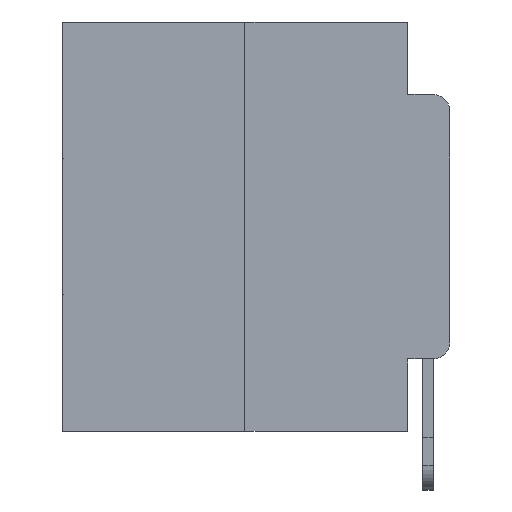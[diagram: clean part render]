
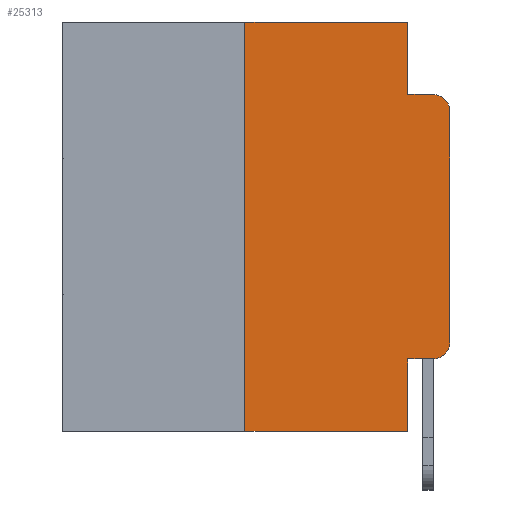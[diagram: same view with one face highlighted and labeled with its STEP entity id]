
A CAD part, left-side view. The second image highlights one B-rep face of the part: STEP entity #25313.
In plain terms, the highlighted planar face has unit normal (-1, 0, 0).
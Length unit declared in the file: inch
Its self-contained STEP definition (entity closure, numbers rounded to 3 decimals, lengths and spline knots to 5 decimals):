
#56 = CARTESIAN_POINT ( 'NONE',  ( 0., 0.25, -0.5 ) ) ;
#1165 = EDGE_CURVE ( 'NONE', #2305, #11096, #11929, .T. ) ;
#1232 = ORIENTED_EDGE ( 'NONE', *, *, #2636, .T. ) ;
#1287 = VECTOR ( 'NONE', #10315, 39.37008 ) ;
#1655 = CARTESIAN_POINT ( 'NONE',  ( 0., 0.051, -0.4115 ) ) ;
#1750 = CARTESIAN_POINT ( 'NONE',  ( 0., 0.051, -0.4115 ) ) ;
#1860 = ORIENTED_EDGE ( 'NONE', *, *, #25212, .T. ) ;
#2025 = AXIS2_PLACEMENT_3D ( 'NONE', #10923, #23818, #4348 ) ;
#2195 = CARTESIAN_POINT ( 'NONE',  ( 0., 0.473, 0. ) ) ;
#2305 = VERTEX_POINT ( 'NONE', #9074 ) ;
#2636 = EDGE_CURVE ( 'NONE', #25847, #20627, #27357, .T. ) ;
#2893 = EDGE_CURVE ( 'NONE', #9911, #21871, #22569, .T. ) ;
#3100 = CARTESIAN_POINT ( 'NONE',  ( 0., 0.02, -0.0885 ) ) ;
#3768 = VECTOR ( 'NONE', #12677, 39.37008 ) ;
#3935 = CARTESIAN_POINT ( 'NONE',  ( 0., 0.051, -0.5 ) ) ;
#4094 = ORIENTED_EDGE ( 'NONE', *, *, #8641, .F. ) ;
#4178 = CARTESIAN_POINT ( 'NONE',  ( 0., 0.051, -0.0885 ) ) ;
#4348 = DIRECTION ( 'NONE',  ( 0., 0., -1. ) ) ;
#4558 = ORIENTED_EDGE ( 'NONE', *, *, #2893, .T. ) ;
#5620 = EDGE_LOOP ( 'NONE', ( #9960, #1232, #25655, #4094, #22461, #27119, #4558, #10765, #1860, #15406 ) ) ;
#5682 = VECTOR ( 'NONE', #23912, 39.37008 ) ;
#6682 = EDGE_CURVE ( 'NONE', #8768, #20627, #23368, .T. ) ;
#6753 = CARTESIAN_POINT ( 'NONE',  ( 0., 0., 0. ) ) ;
#7054 = DIRECTION ( 'NONE',  ( 0., 0., -1. ) ) ;
#7093 = EDGE_CURVE ( 'NONE', #20883, #25847, #18892, .T. ) ;
#7297 = DIRECTION ( 'NONE',  ( 0., -1., 0. ) ) ;
#7792 = CARTESIAN_POINT ( 'NONE',  ( 0., 0.051, 0. ) ) ;
#7895 = FACE_OUTER_BOUND ( 'NONE', #5620, .T. ) ;
#8641 = EDGE_CURVE ( 'NONE', #11096, #8768, #22210, .T. ) ;
#8768 = VERTEX_POINT ( 'NONE', #4178 ) ;
#9074 = CARTESIAN_POINT ( 'NONE',  ( 0., 0.25, 0. ) ) ;
#9911 = VERTEX_POINT ( 'NONE', #56 ) ;
#9960 = ORIENTED_EDGE ( 'NONE', *, *, #7093, .T. ) ;
#10315 = DIRECTION ( 'NONE',  ( 0., -1., 0. ) ) ;
#10755 = DIRECTION ( 'NONE',  ( 0., 0., -1. ) ) ;
#10765 = ORIENTED_EDGE ( 'NONE', *, *, #27550, .F. ) ;
#10923 = CARTESIAN_POINT ( 'NONE',  ( 0., 0.02, -0.1085 ) ) ;
#11096 = VERTEX_POINT ( 'NONE', #12722 ) ;
#11775 = LINE ( 'NONE', #24078, #27064 ) ;
#11929 = LINE ( 'NONE', #18627, #14649 ) ;
#11993 = VERTEX_POINT ( 'NONE', #12657 ) ;
#12657 = CARTESIAN_POINT ( 'NONE',  ( 0., 0.02, -0.4115 ) ) ;
#12677 = DIRECTION ( 'NONE',  ( 0., -1., 0. ) ) ;
#12722 = CARTESIAN_POINT ( 'NONE',  ( 0., 0.051, 0. ) ) ;
#12748 = CARTESIAN_POINT ( 'NONE',  ( 0., 0.051, 0. ) ) ;
#13076 = VECTOR ( 'NONE', #7297, 39.37008 ) ;
#13305 = AXIS2_PLACEMENT_3D ( 'NONE', #20034, #20320, #7054 ) ;
#13353 = AXIS2_PLACEMENT_3D ( 'NONE', #2195, #23748, #10755 ) ;
#13479 = EDGE_CURVE ( 'NONE', #11993, #20883, #24981, .T. ) ;
#14649 = VECTOR ( 'NONE', #18724, 39.37008 ) ;
#14951 = CARTESIAN_POINT ( 'NONE',  ( 0., 0.051, -0.0885 ) ) ;
#15406 = ORIENTED_EDGE ( 'NONE', *, *, #13479, .T. ) ;
#16111 = VERTEX_POINT ( 'NONE', #1655 ) ;
#18627 = CARTESIAN_POINT ( 'NONE',  ( 0., 0.473, 0. ) ) ;
#18724 = DIRECTION ( 'NONE',  ( 0., -1., 0. ) ) ;
#18892 = LINE ( 'NONE', #6753, #5682 ) ;
#19510 = EDGE_CURVE ( 'NONE', #9911, #2305, #11775, .T. ) ;
#20034 = CARTESIAN_POINT ( 'NONE',  ( 0., 0.02, -0.3915 ) ) ;
#20320 = DIRECTION ( 'NONE',  ( -1., 0., 0. ) ) ;
#20396 = VECTOR ( 'NONE', #27342, 39.37008 ) ;
#20473 = CARTESIAN_POINT ( 'NONE',  ( 0., 0.473, -0.5 ) ) ;
#20627 = VERTEX_POINT ( 'NONE', #3100 ) ;
#20883 = VERTEX_POINT ( 'NONE', #23564 ) ;
#21242 = CARTESIAN_POINT ( 'NONE',  ( 0., 0., -0.1085 ) ) ;
#21470 = PLANE ( 'NONE',  #13353 ) ;
#21871 = VERTEX_POINT ( 'NONE', #3935 ) ;
#21970 = DIRECTION ( 'NONE',  ( 0., 0., 1. ) ) ;
#22210 = LINE ( 'NONE', #12748, #26628 ) ;
#22461 = ORIENTED_EDGE ( 'NONE', *, *, #1165, .F. ) ;
#22569 = LINE ( 'NONE', #20473, #13076 ) ;
#23368 = LINE ( 'NONE', #14951, #1287 ) ;
#23564 = CARTESIAN_POINT ( 'NONE',  ( 0., 0., -0.3915 ) ) ;
#23640 = DIRECTION ( 'NONE',  ( 0., 0., -1. ) ) ;
#23748 = DIRECTION ( 'NONE',  ( 1., 0., 0. ) ) ;
#23818 = DIRECTION ( 'NONE',  ( -1., 0., 0. ) ) ;
#23912 = DIRECTION ( 'NONE',  ( 0., 0., 1. ) ) ;
#24078 = CARTESIAN_POINT ( 'NONE',  ( 0., 0.25, 0. ) ) ;
#24981 = CIRCLE ( 'NONE', #13305, 0.02 ) ;
#25212 = EDGE_CURVE ( 'NONE', #16111, #11993, #26889, .T. ) ;
#25313 = ADVANCED_FACE ( 'NONE', ( #7895 ), #21470, .F. ) ;
#25655 = ORIENTED_EDGE ( 'NONE', *, *, #6682, .F. ) ;
#25847 = VERTEX_POINT ( 'NONE', #21242 ) ;
#26628 = VECTOR ( 'NONE', #23640, 39.37008 ) ;
#26889 = LINE ( 'NONE', #1750, #3768 ) ;
#27064 = VECTOR ( 'NONE', #21970, 39.37008 ) ;
#27119 = ORIENTED_EDGE ( 'NONE', *, *, #19510, .F. ) ;
#27342 = DIRECTION ( 'NONE',  ( 0., 0., -1. ) ) ;
#27357 = CIRCLE ( 'NONE', #2025, 0.02 ) ;
#27550 = EDGE_CURVE ( 'NONE', #16111, #21871, #27940, .T. ) ;
#27940 = LINE ( 'NONE', #7792, #20396 ) ;
